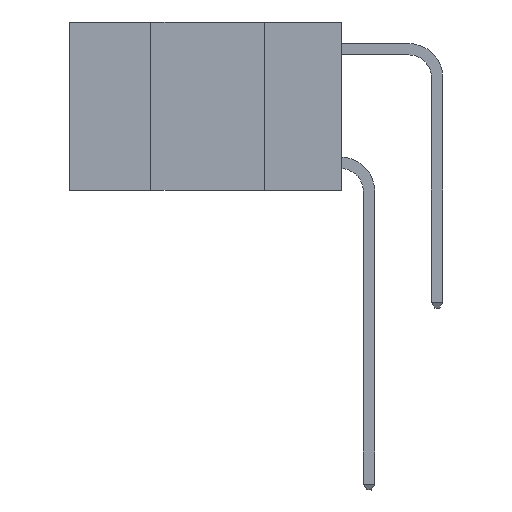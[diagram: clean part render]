
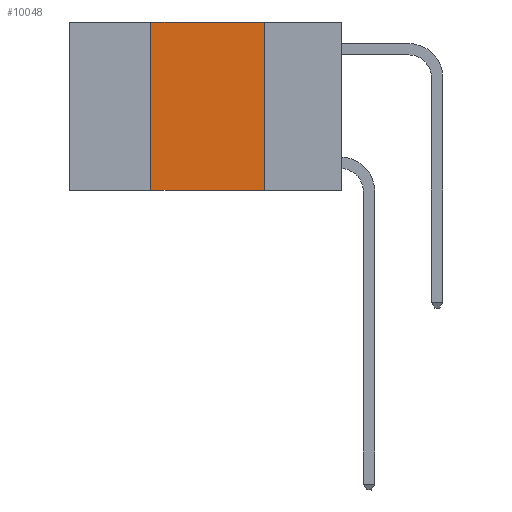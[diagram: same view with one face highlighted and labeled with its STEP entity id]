
A CAD part, left-side view. The second image highlights one B-rep face of the part: STEP entity #10048.
In plain terms, the highlighted planar face has unit normal (-1, 0, 0).
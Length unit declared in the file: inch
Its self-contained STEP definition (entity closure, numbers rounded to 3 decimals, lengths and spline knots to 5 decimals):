
#58 = LINE ( 'NONE', #8130, #25357 ) ;
#1059 = PLANE ( 'NONE',  #25543 ) ;
#2753 = FACE_OUTER_BOUND ( 'NONE', #18249, .T. ) ;
#2840 = EDGE_CURVE ( 'NONE', #7785, #11646, #7727, .T. ) ;
#2881 = VECTOR ( 'NONE', #17274, 39.37008 ) ;
#3061 = ORIENTED_EDGE ( 'NONE', *, *, #14682, .T. ) ;
#3660 = VERTEX_POINT ( 'NONE', #4367 ) ;
#3864 = CARTESIAN_POINT ( 'NONE',  ( 0., 0.42, -0.37 ) ) ;
#4329 = CARTESIAN_POINT ( 'NONE',  ( 0., 0.42, 0. ) ) ;
#4367 = CARTESIAN_POINT ( 'NONE',  ( 0., 0.17, -0.37 ) ) ;
#6558 = EDGE_CURVE ( 'NONE', #8494, #7785, #58, .T. ) ;
#7494 = DIRECTION ( 'NONE',  ( 0., -1., 0. ) ) ;
#7727 = LINE ( 'NONE', #25455, #2881 ) ;
#7785 = VERTEX_POINT ( 'NONE', #4329 ) ;
#8130 = CARTESIAN_POINT ( 'NONE',  ( 0., 0.42, 0. ) ) ;
#8494 = VERTEX_POINT ( 'NONE', #3864 ) ;
#10020 = LINE ( 'NONE', #12484, #10185 ) ;
#10048 = ADVANCED_FACE ( 'NONE', ( #2753 ), #1059, .F. ) ;
#10185 = VECTOR ( 'NONE', #12343, 39.37008 ) ;
#11123 = ORIENTED_EDGE ( 'NONE', *, *, #6558, .F. ) ;
#11646 = VERTEX_POINT ( 'NONE', #19528 ) ;
#12343 = DIRECTION ( 'NONE',  ( 0., 0., -1. ) ) ;
#12484 = CARTESIAN_POINT ( 'NONE',  ( 0., 0.17, 0. ) ) ;
#13056 = DIRECTION ( 'NONE',  ( 1., 0., 0. ) ) ;
#14682 = EDGE_CURVE ( 'NONE', #8494, #3660, #19502, .T. ) ;
#15030 = CARTESIAN_POINT ( 'NONE',  ( 0., 0.6, 0. ) ) ;
#17274 = DIRECTION ( 'NONE',  ( 0., -1., 0. ) ) ;
#18249 = EDGE_LOOP ( 'NONE', ( #22534, #22292, #11123, #3061 ) ) ;
#18632 = EDGE_CURVE ( 'NONE', #11646, #3660, #10020, .T. ) ;
#19502 = LINE ( 'NONE', #21080, #21064 ) ;
#19528 = CARTESIAN_POINT ( 'NONE',  ( 0., 0.17, 0. ) ) ;
#21032 = DIRECTION ( 'NONE',  ( 0., 0., -1. ) ) ;
#21064 = VECTOR ( 'NONE', #7494, 39.37008 ) ;
#21080 = CARTESIAN_POINT ( 'NONE',  ( 0., 0.6, -0.37 ) ) ;
#22292 = ORIENTED_EDGE ( 'NONE', *, *, #2840, .F. ) ;
#22534 = ORIENTED_EDGE ( 'NONE', *, *, #18632, .F. ) ;
#24451 = DIRECTION ( 'NONE',  ( 0., 0., 1. ) ) ;
#25357 = VECTOR ( 'NONE', #24451, 39.37008 ) ;
#25455 = CARTESIAN_POINT ( 'NONE',  ( 0., 0.6, 0. ) ) ;
#25543 = AXIS2_PLACEMENT_3D ( 'NONE', #15030, #13056, #21032 ) ;
